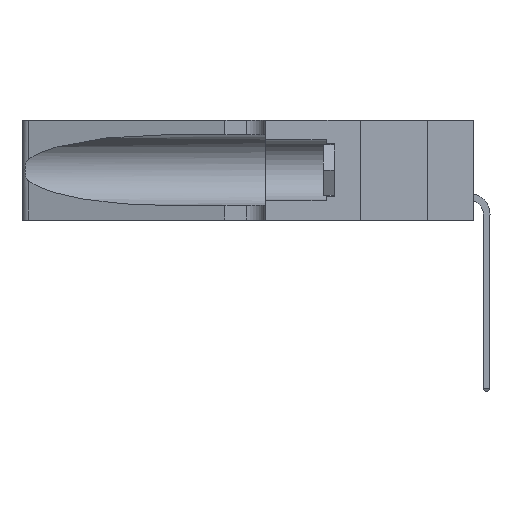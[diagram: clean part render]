
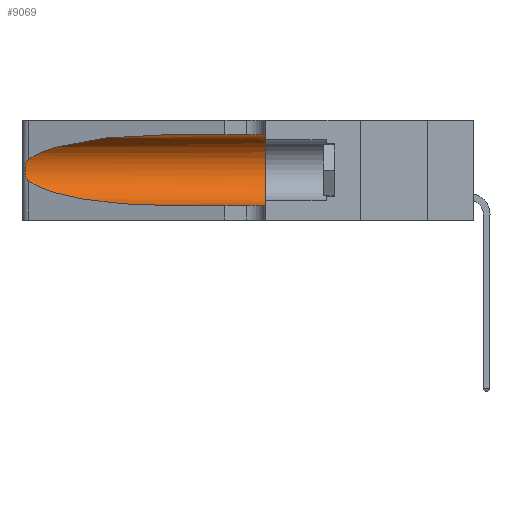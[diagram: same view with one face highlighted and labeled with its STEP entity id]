
A CAD part, left-side view. The second image highlights one B-rep face of the part: STEP entity #9069.
In plain terms, the highlighted cylindrical face has radius 3.308 mm (diameter 6.617 mm), a partial arc.
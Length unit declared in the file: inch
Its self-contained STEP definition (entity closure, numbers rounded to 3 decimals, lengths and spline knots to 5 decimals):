
#174 = EDGE_LOOP ( 'NONE', ( #5936, #10545, #19483, #34784, #17895, #35345 ) ) ;
#1095 = CARTESIAN_POINT ( 'NONE',  ( 0.25787, 1.23484, 0.2124 ) ) ;
#1171 = EDGE_CURVE ( 'NONE', #35503, #22258, #40605, .T. ) ;
#3048 = EDGE_CURVE ( 'NONE', #32655, #28748, #8756, .T. ) ;
#3117 = DIRECTION ( 'NONE',  ( 0., 0., 1. ) ) ;
#3329 = CARTESIAN_POINT ( 'NONE',  ( 0.1305, 1.61858, 0.31525 ) ) ;
#3792 = DIRECTION ( 'NONE',  ( 0., -1., 0. ) ) ;
#4018 = EDGE_CURVE ( 'NONE', #32849, #23748, #6465, .T. ) ;
#4371 = CARTESIAN_POINT ( 'NONE',  ( 0.2373, 1.15595, 0.28018 ) ) ;
#5936 = ORIENTED_EDGE ( 'NONE', *, *, #4018, .T. ) ;
#6465 =( BOUNDED_CURVE ( )  B_SPLINE_CURVE ( 3, ( #13871, #20289, #4371, #13473 ),
 .UNSPECIFIED., .F., .T. ) 
 B_SPLINE_CURVE_WITH_KNOTS ( ( 4, 4 ),
 ( 1.5708, 2.84003 ),
 .UNSPECIFIED. ) 
 CURVE ( )  GEOMETRIC_REPRESENTATION_ITEM ( )  RATIONAL_B_SPLINE_CURVE ( ( 1., 0.87, 0.87, 1. ) ) 
 REPRESENTATION_ITEM ( '' )  );
#8110 = CARTESIAN_POINT ( 'NONE',  ( 0.25789, 1.23486, 0.15765 ) ) ;
#8756 =( BOUNDED_CURVE ( )  B_SPLINE_CURVE ( 3, ( #12427, #37683, #24965, #18220 ),
 .UNSPECIFIED., .F., .T. ) 
 B_SPLINE_CURVE_WITH_KNOTS ( ( 4, 4 ),
 ( 3.44316, 4.71239 ),
 .UNSPECIFIED. ) 
 CURVE ( )  GEOMETRIC_REPRESENTATION_ITEM ( )  RATIONAL_B_SPLINE_CURVE ( ( 1., 0.87, 0.87, 1. ) ) 
 REPRESENTATION_ITEM ( '' )  );
#9069 = ADVANCED_FACE ( 'NONE', ( #9104 ), #37051, .F. ) ;
#9104 = FACE_OUTER_BOUND ( 'NONE', #174, .T. ) ;
#10545 = ORIENTED_EDGE ( 'NONE', *, *, #19681, .T. ) ;
#11582 = EDGE_CURVE ( 'NONE', #28748, #22258, #26749, .T. ) ;
#11767 = LINE ( 'NONE', #3329, #17217 ) ;
#11977 = DIRECTION ( 'NONE',  ( 0., 0., -1. ) ) ;
#12035 = CARTESIAN_POINT ( 'NONE',  ( 0.1305, 0.35, 0.185 ) ) ;
#12427 = CARTESIAN_POINT ( 'NONE',  ( 0.25487, 1.22718, 0.14631 ) ) ;
#12893 = CARTESIAN_POINT ( 'NONE',  ( 0.25487, 1.22718, 0.14631 ) ) ;
#13391 = CARTESIAN_POINT ( 'NONE',  ( 0.25487, 1.22718, 0.22369 ) ) ;
#13473 = CARTESIAN_POINT ( 'NONE',  ( 0.25487, 1.22718, 0.22369 ) ) ;
#13871 = CARTESIAN_POINT ( 'NONE',  ( 0.1305, 0.72297, 0.31525 ) ) ;
#14126 = CARTESIAN_POINT ( 'NONE',  ( 0.25555, 1.22994, 0.2215 ) ) ;
#14320 = EDGE_CURVE ( 'NONE', #32849, #35503, #11767, .T. ) ;
#14414 = CARTESIAN_POINT ( 'NONE',  ( 0.25487, 1.22718, 0.22369 ) ) ;
#15327 = CARTESIAN_POINT ( 'NONE',  ( 0.1305, 1.61858, 0.185 ) ) ;
#16209 = B_SPLINE_CURVE_WITH_KNOTS ( 'NONE', 3,
 ( #14414, #14126, #33128, #1095, #39948, #36907, #30156, #27227, #17192, #39533, #8110, #39380, #20269, #23760 ),
 .UNSPECIFIED., .F., .F.,
 ( 4, 2, 2, 2, 2, 2, 4 ),
 ( 0., 0.00027, 0.00053, 0.00107, 0.0016, 0.00187, 0.00214 ),
 .UNSPECIFIED. ) ;
#17192 = CARTESIAN_POINT ( 'NONE',  ( 0.26017, 1.23833, 0.17102 ) ) ;
#17217 = VECTOR ( 'NONE', #3792, 39.37008 ) ;
#17395 = CARTESIAN_POINT ( 'NONE',  ( 0.1305, 0.35, 0.05475 ) ) ;
#17733 = CARTESIAN_POINT ( 'NONE',  ( 0.1305, 0.72297, 0.05475 ) ) ;
#17895 = ORIENTED_EDGE ( 'NONE', *, *, #1171, .F. ) ;
#18220 = CARTESIAN_POINT ( 'NONE',  ( 0.1305, 0.72297, 0.05475 ) ) ;
#19483 = ORIENTED_EDGE ( 'NONE', *, *, #3048, .T. ) ;
#19681 = EDGE_CURVE ( 'NONE', #23748, #32655, #16209, .T. ) ;
#20269 = CARTESIAN_POINT ( 'NONE',  ( 0.25555, 1.22993, 0.14849 ) ) ;
#20289 = CARTESIAN_POINT ( 'NONE',  ( 0.18966, 0.96281, 0.31525 ) ) ;
#20628 = CARTESIAN_POINT ( 'NONE',  ( 0.1305, 1.61858, 0.05475 ) ) ;
#22258 = VERTEX_POINT ( 'NONE', #17395 ) ;
#23748 = VERTEX_POINT ( 'NONE', #13391 ) ;
#23760 = CARTESIAN_POINT ( 'NONE',  ( 0.25487, 1.22718, 0.14631 ) ) ;
#23839 = AXIS2_PLACEMENT_3D ( 'NONE', #15327, #40711, #11977 ) ;
#24842 = DIRECTION ( 'NONE',  ( 0., -1., 0. ) ) ;
#24965 = CARTESIAN_POINT ( 'NONE',  ( 0.18966, 0.96281, 0.05475 ) ) ;
#25458 = AXIS2_PLACEMENT_3D ( 'NONE', #12035, #37585, #3117 ) ;
#26749 = LINE ( 'NONE', #20628, #41367 ) ;
#27227 = CARTESIAN_POINT ( 'NONE',  ( 0.26075, 1.23896, 0.178 ) ) ;
#28748 = VERTEX_POINT ( 'NONE', #17733 ) ;
#30156 = CARTESIAN_POINT ( 'NONE',  ( 0.26075, 1.23896, 0.19203 ) ) ;
#32655 = VERTEX_POINT ( 'NONE', #12893 ) ;
#32849 = VERTEX_POINT ( 'NONE', #36589 ) ;
#33128 = CARTESIAN_POINT ( 'NONE',  ( 0.25639, 1.23184, 0.21858 ) ) ;
#34784 = ORIENTED_EDGE ( 'NONE', *, *, #11582, .T. ) ;
#35345 = ORIENTED_EDGE ( 'NONE', *, *, #14320, .F. ) ;
#35503 = VERTEX_POINT ( 'NONE', #40513 ) ;
#36589 = CARTESIAN_POINT ( 'NONE',  ( 0.1305, 0.72297, 0.31525 ) ) ;
#36907 = CARTESIAN_POINT ( 'NONE',  ( 0.26018, 1.23835, 0.19895 ) ) ;
#37051 = CYLINDRICAL_SURFACE ( 'NONE', #23839, 0.13025 ) ;
#37585 = DIRECTION ( 'NONE',  ( 0., 1., 0. ) ) ;
#37683 = CARTESIAN_POINT ( 'NONE',  ( 0.2373, 1.15595, 0.08982 ) ) ;
#39380 = CARTESIAN_POINT ( 'NONE',  ( 0.25639, 1.23186, 0.15144 ) ) ;
#39533 = CARTESIAN_POINT ( 'NONE',  ( 0.25856, 1.23593, 0.16098 ) ) ;
#39948 = CARTESIAN_POINT ( 'NONE',  ( 0.25854, 1.2359, 0.20912 ) ) ;
#40513 = CARTESIAN_POINT ( 'NONE',  ( 0.1305, 0.35, 0.31525 ) ) ;
#40605 = CIRCLE ( 'NONE', #25458, 0.13025 ) ;
#40711 = DIRECTION ( 'NONE',  ( 0., -1., 0. ) ) ;
#41367 = VECTOR ( 'NONE', #24842, 39.37008 ) ;
